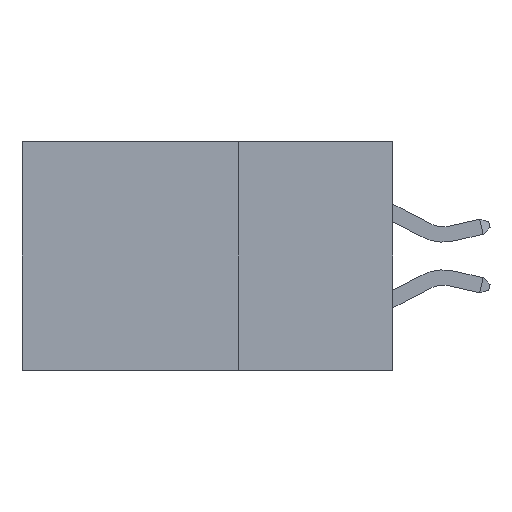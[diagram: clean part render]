
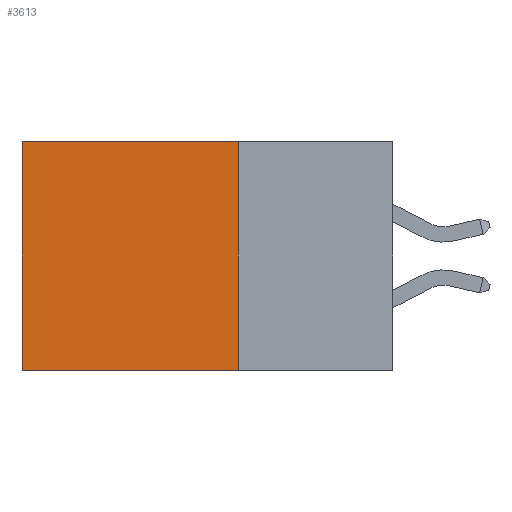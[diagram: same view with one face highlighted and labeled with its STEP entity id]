
A CAD part, left-side view. The second image highlights one B-rep face of the part: STEP entity #3613.
In plain terms, the highlighted planar face has unit normal (-1, 0, 0).
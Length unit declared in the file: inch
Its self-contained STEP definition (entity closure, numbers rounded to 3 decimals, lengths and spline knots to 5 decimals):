
#912 = DIRECTION ( 'NONE',  ( 0., 1., 0. ) ) ;
#1209 = DIRECTION ( 'NONE',  ( 0., 0., -1. ) ) ;
#1371 = PLANE ( 'NONE',  #2112 ) ;
#2112 = AXIS2_PLACEMENT_3D ( 'NONE', #19670, #4902, #1209 ) ;
#3031 = CARTESIAN_POINT ( 'NONE',  ( 0.2875, 0.25, 0. ) ) ;
#3613 = ADVANCED_FACE ( 'NONE', ( #22592 ), #1371, .F. ) ;
#4468 = EDGE_CURVE ( 'NONE', #7240, #12419, #15657, .T. ) ;
#4902 = DIRECTION ( 'NONE',  ( 1., 0., 0. ) ) ;
#5312 = ORIENTED_EDGE ( 'NONE', *, *, #4468, .T. ) ;
#6111 = ORIENTED_EDGE ( 'NONE', *, *, #13815, .F. ) ;
#6243 = ORIENTED_EDGE ( 'NONE', *, *, #9561, .T. ) ;
#6824 = LINE ( 'NONE', #3031, #12930 ) ;
#7226 = CARTESIAN_POINT ( 'NONE',  ( 0.2875, 0.6, 0. ) ) ;
#7240 = VERTEX_POINT ( 'NONE', #11211 ) ;
#7242 = VECTOR ( 'NONE', #11888, 39.37008 ) ;
#7276 = DIRECTION ( 'NONE',  ( 0., 0., -1. ) ) ;
#9561 = EDGE_CURVE ( 'NONE', #11633, #7240, #6824, .T. ) ;
#9597 = CARTESIAN_POINT ( 'NONE',  ( 0.2875, 0.6, -0.37 ) ) ;
#10137 = VECTOR ( 'NONE', #7276, 39.37008 ) ;
#11211 = CARTESIAN_POINT ( 'NONE',  ( 0.2875, 0.6, 0. ) ) ;
#11633 = VERTEX_POINT ( 'NONE', #23059 ) ;
#11888 = DIRECTION ( 'NONE',  ( 0., 1., 0. ) ) ;
#12419 = VERTEX_POINT ( 'NONE', #9597 ) ;
#12930 = VECTOR ( 'NONE', #912, 39.37008 ) ;
#13815 = EDGE_CURVE ( 'NONE', #21474, #12419, #18295, .T. ) ;
#14878 = EDGE_LOOP ( 'NONE', ( #5312, #6111, #17891, #6243 ) ) ;
#14999 = CARTESIAN_POINT ( 'NONE',  ( 0.2875, 0.25, -0.37 ) ) ;
#15093 = LINE ( 'NONE', #22193, #10137 ) ;
#15657 = LINE ( 'NONE', #7226, #19423 ) ;
#17891 = ORIENTED_EDGE ( 'NONE', *, *, #19346, .F. ) ;
#18295 = LINE ( 'NONE', #22829, #7242 ) ;
#18475 = DIRECTION ( 'NONE',  ( 0., 0., -1. ) ) ;
#19346 = EDGE_CURVE ( 'NONE', #11633, #21474, #15093, .T. ) ;
#19423 = VECTOR ( 'NONE', #18475, 39.37008 ) ;
#19670 = CARTESIAN_POINT ( 'NONE',  ( 0.2875, 0.25, 0. ) ) ;
#21474 = VERTEX_POINT ( 'NONE', #14999 ) ;
#22193 = CARTESIAN_POINT ( 'NONE',  ( 0.2875, 0.25, 0. ) ) ;
#22592 = FACE_OUTER_BOUND ( 'NONE', #14878, .T. ) ;
#22829 = CARTESIAN_POINT ( 'NONE',  ( 0.2875, 0.25, -0.37 ) ) ;
#23059 = CARTESIAN_POINT ( 'NONE',  ( 0.2875, 0.25, 0. ) ) ;
